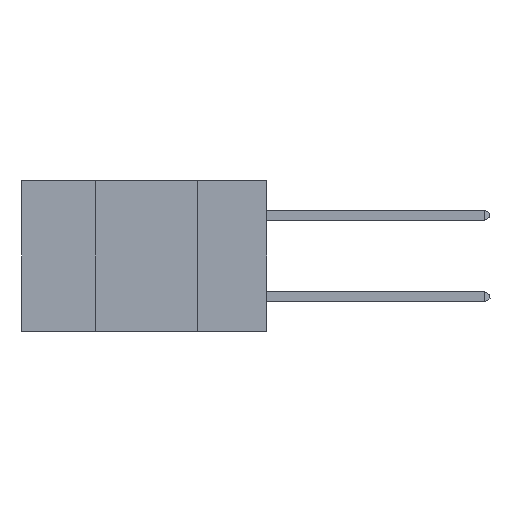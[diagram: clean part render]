
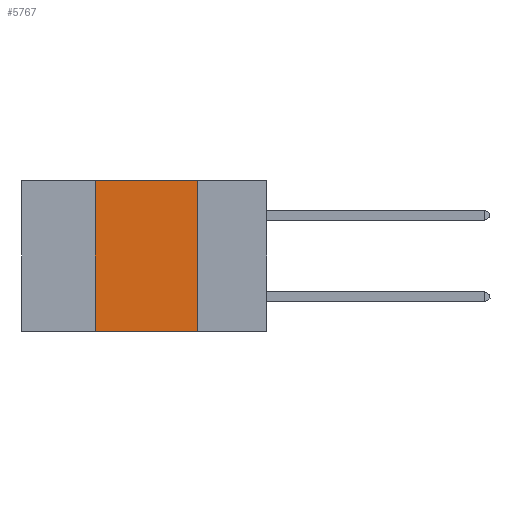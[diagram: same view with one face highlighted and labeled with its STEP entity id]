
A CAD part, left-side view. The second image highlights one B-rep face of the part: STEP entity #5767.
In plain terms, the highlighted planar face has unit normal (-1, 0, 0).
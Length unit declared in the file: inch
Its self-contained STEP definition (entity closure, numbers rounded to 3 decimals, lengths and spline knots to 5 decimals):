
#414 = DIRECTION ( 'NONE',  ( 0., 0., -1. ) ) ;
#474 = CARTESIAN_POINT ( 'NONE',  ( 0., 0.17, 0. ) ) ;
#732 = CARTESIAN_POINT ( 'NONE',  ( 0., 0.6, 0. ) ) ;
#1721 = CARTESIAN_POINT ( 'NONE',  ( 0., 0.42, 0. ) ) ;
#2123 = DIRECTION ( 'NONE',  ( 0., -1., 0. ) ) ;
#3284 = ORIENTED_EDGE ( 'NONE', *, *, #6381, .F. ) ;
#3365 = FACE_OUTER_BOUND ( 'NONE', #9455, .T. ) ;
#3789 = EDGE_CURVE ( 'NONE', #7934, #15626, #8816, .T. ) ;
#3903 = CARTESIAN_POINT ( 'NONE',  ( 0., 0.42, 0. ) ) ;
#4147 = LINE ( 'NONE', #12441, #7135 ) ;
#4731 = PLANE ( 'NONE',  #8593 ) ;
#4739 = LINE ( 'NONE', #732, #10854 ) ;
#5402 = ORIENTED_EDGE ( 'NONE', *, *, #3789, .F. ) ;
#5513 = EDGE_CURVE ( 'NONE', #11821, #16442, #11711, .T. ) ;
#5767 = ADVANCED_FACE ( 'NONE', ( #3365 ), #4731, .F. ) ;
#6381 = EDGE_CURVE ( 'NONE', #16442, #7934, #4739, .T. ) ;
#6999 = EDGE_CURVE ( 'NONE', #11821, #15626, #4147, .T. ) ;
#7135 = VECTOR ( 'NONE', #8537, 39.37008 ) ;
#7362 = DIRECTION ( 'NONE',  ( 1., 0., 0. ) ) ;
#7934 = VERTEX_POINT ( 'NONE', #7972 ) ;
#7972 = CARTESIAN_POINT ( 'NONE',  ( 0., 0.17, 0. ) ) ;
#8537 = DIRECTION ( 'NONE',  ( 0., -1., 0. ) ) ;
#8593 = AXIS2_PLACEMENT_3D ( 'NONE', #11303, #7362, #16430 ) ;
#8816 = LINE ( 'NONE', #474, #11929 ) ;
#9455 = EDGE_LOOP ( 'NONE', ( #5402, #3284, #14311, #16627 ) ) ;
#9505 = DIRECTION ( 'NONE',  ( 0., 0., 1. ) ) ;
#10854 = VECTOR ( 'NONE', #2123, 39.37008 ) ;
#11277 = CARTESIAN_POINT ( 'NONE',  ( 0., 0.42, -0.37 ) ) ;
#11303 = CARTESIAN_POINT ( 'NONE',  ( 0., 0.6, 0. ) ) ;
#11427 = CARTESIAN_POINT ( 'NONE',  ( 0., 0.17, -0.37 ) ) ;
#11711 = LINE ( 'NONE', #1721, #15094 ) ;
#11821 = VERTEX_POINT ( 'NONE', #11277 ) ;
#11929 = VECTOR ( 'NONE', #414, 39.37008 ) ;
#12441 = CARTESIAN_POINT ( 'NONE',  ( 0., 0.6, -0.37 ) ) ;
#14311 = ORIENTED_EDGE ( 'NONE', *, *, #5513, .F. ) ;
#15094 = VECTOR ( 'NONE', #9505, 39.37008 ) ;
#15626 = VERTEX_POINT ( 'NONE', #11427 ) ;
#16430 = DIRECTION ( 'NONE',  ( 0., 0., -1. ) ) ;
#16442 = VERTEX_POINT ( 'NONE', #3903 ) ;
#16627 = ORIENTED_EDGE ( 'NONE', *, *, #6999, .T. ) ;
